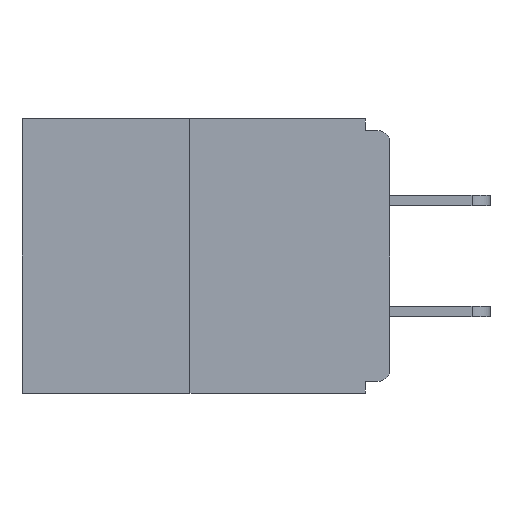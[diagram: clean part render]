
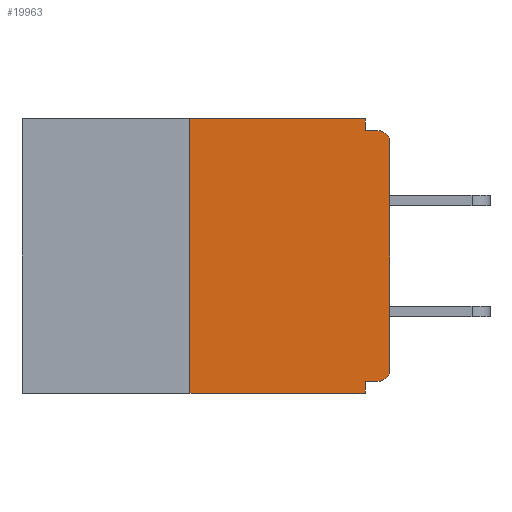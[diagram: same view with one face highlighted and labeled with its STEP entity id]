
A CAD part, left-side view. The second image highlights one B-rep face of the part: STEP entity #19963.
In plain terms, the highlighted planar face has unit normal (-1, 0, 0).
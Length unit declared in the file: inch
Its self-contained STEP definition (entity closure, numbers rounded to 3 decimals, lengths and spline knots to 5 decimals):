
#138 = LINE ( 'NONE', #4643, #24657 ) ;
#224 = AXIS2_PLACEMENT_3D ( 'NONE', #18330, #16523, #4364 ) ;
#306 = CARTESIAN_POINT ( 'NONE',  ( 0., 0.015, -0.015 ) ) ;
#425 = VECTOR ( 'NONE', #6762, 39.37008 ) ;
#967 = CARTESIAN_POINT ( 'NONE',  ( 0., 0.031, 0. ) ) ;
#1946 = AXIS2_PLACEMENT_3D ( 'NONE', #11860, #19660, #15845 ) ;
#2314 = VECTOR ( 'NONE', #6953, 39.37008 ) ;
#3305 = CIRCLE ( 'NONE', #224, 0.015 ) ;
#3632 = CARTESIAN_POINT ( 'NONE',  ( 0., 0.25, 0. ) ) ;
#3695 = VERTEX_POINT ( 'NONE', #3632 ) ;
#3914 = CARTESIAN_POINT ( 'NONE',  ( 0., 0.015, -0.328 ) ) ;
#3977 = EDGE_CURVE ( 'NONE', #23611, #12192, #20432, .T. ) ;
#4364 = DIRECTION ( 'NONE',  ( 0., 0., -1. ) ) ;
#4429 = ORIENTED_EDGE ( 'NONE', *, *, #24929, .F. ) ;
#4643 = CARTESIAN_POINT ( 'NONE',  ( 0., 0., -0.015 ) ) ;
#5482 = CARTESIAN_POINT ( 'NONE',  ( 0., 0.031, -0.015 ) ) ;
#5668 = EDGE_LOOP ( 'NONE', ( #17710, #5716, #22383, #4429, #19075, #8881, #5933, #19249, #15298, #19998 ) ) ;
#5716 = ORIENTED_EDGE ( 'NONE', *, *, #23115, .F. ) ;
#5933 = ORIENTED_EDGE ( 'NONE', *, *, #22079, .T. ) ;
#5992 = EDGE_CURVE ( 'NONE', #10187, #15060, #15591, .T. ) ;
#6681 = DIRECTION ( 'NONE',  ( 0., -1., 0. ) ) ;
#6762 = DIRECTION ( 'NONE',  ( 0., -1., 0. ) ) ;
#6953 = DIRECTION ( 'NONE',  ( 0., 1., 0. ) ) ;
#7119 = LINE ( 'NONE', #25156, #425 ) ;
#8229 = DIRECTION ( 'NONE',  ( -1., 0., 0. ) ) ;
#8346 = FACE_OUTER_BOUND ( 'NONE', #5668, .T. ) ;
#8674 = DIRECTION ( 'NONE',  ( 0., 0., 1. ) ) ;
#8881 = ORIENTED_EDGE ( 'NONE', *, *, #19013, .T. ) ;
#8905 = CARTESIAN_POINT ( 'NONE',  ( 0., 0., -0.328 ) ) ;
#9274 = CARTESIAN_POINT ( 'NONE',  ( 0., 0., -0.03 ) ) ;
#10022 = CARTESIAN_POINT ( 'NONE',  ( 0., 0.25, -0.343 ) ) ;
#10187 = VERTEX_POINT ( 'NONE', #9274 ) ;
#10892 = EDGE_CURVE ( 'NONE', #13697, #20250, #13803, .T. ) ;
#11008 = CARTESIAN_POINT ( 'NONE',  ( 0., 0., 0. ) ) ;
#11817 = CARTESIAN_POINT ( 'NONE',  ( 0., 0.031, 0. ) ) ;
#11860 = CARTESIAN_POINT ( 'NONE',  ( 0., 0.46, 0. ) ) ;
#12050 = VECTOR ( 'NONE', #12656, 39.37008 ) ;
#12128 = AXIS2_PLACEMENT_3D ( 'NONE', #18257, #8229, #24152 ) ;
#12192 = VERTEX_POINT ( 'NONE', #5482 ) ;
#12656 = DIRECTION ( 'NONE',  ( 0., 0., 1. ) ) ;
#13367 = VECTOR ( 'NONE', #8674, 39.37008 ) ;
#13697 = VERTEX_POINT ( 'NONE', #3914 ) ;
#13698 = PLANE ( 'NONE',  #1946 ) ;
#13803 = LINE ( 'NONE', #8905, #2314 ) ;
#15060 = VERTEX_POINT ( 'NONE', #306 ) ;
#15298 = ORIENTED_EDGE ( 'NONE', *, *, #26276, .F. ) ;
#15591 = CIRCLE ( 'NONE', #12128, 0.015 ) ;
#15766 = VECTOR ( 'NONE', #22341, 39.37008 ) ;
#15845 = DIRECTION ( 'NONE',  ( 0., 0., -1. ) ) ;
#16206 = LINE ( 'NONE', #11008, #13367 ) ;
#16388 = LINE ( 'NONE', #24150, #15766 ) ;
#16523 = DIRECTION ( 'NONE',  ( -1., 0., 0. ) ) ;
#16719 = CARTESIAN_POINT ( 'NONE',  ( 0., 0.25, 0. ) ) ;
#17710 = ORIENTED_EDGE ( 'NONE', *, *, #19115, .F. ) ;
#18257 = CARTESIAN_POINT ( 'NONE',  ( 0., 0.015, -0.03 ) ) ;
#18330 = CARTESIAN_POINT ( 'NONE',  ( 0., 0.015, -0.313 ) ) ;
#18828 = CARTESIAN_POINT ( 'NONE',  ( 0., 0.031, -0.343 ) ) ;
#19013 = EDGE_CURVE ( 'NONE', #13697, #20844, #3305, .T. ) ;
#19042 = CARTESIAN_POINT ( 'NONE',  ( 0., 0., -0.313 ) ) ;
#19075 = ORIENTED_EDGE ( 'NONE', *, *, #10892, .F. ) ;
#19115 = EDGE_CURVE ( 'NONE', #3695, #23611, #7119, .T. ) ;
#19249 = ORIENTED_EDGE ( 'NONE', *, *, #5992, .T. ) ;
#19660 = DIRECTION ( 'NONE',  ( 1., 0., 0. ) ) ;
#19792 = VECTOR ( 'NONE', #24338, 39.37008 ) ;
#19963 = ADVANCED_FACE ( 'NONE', ( #8346 ), #13698, .F. ) ;
#19998 = ORIENTED_EDGE ( 'NONE', *, *, #3977, .F. ) ;
#20250 = VERTEX_POINT ( 'NONE', #22997 ) ;
#20432 = LINE ( 'NONE', #11817, #19792 ) ;
#20664 = VERTEX_POINT ( 'NONE', #10022 ) ;
#20844 = VERTEX_POINT ( 'NONE', #19042 ) ;
#20860 = VECTOR ( 'NONE', #21722, 39.37008 ) ;
#21722 = DIRECTION ( 'NONE',  ( 0., -1., 0. ) ) ;
#22079 = EDGE_CURVE ( 'NONE', #20844, #10187, #16206, .T. ) ;
#22341 = DIRECTION ( 'NONE',  ( 0., 0., -1. ) ) ;
#22383 = ORIENTED_EDGE ( 'NONE', *, *, #24678, .T. ) ;
#22835 = LINE ( 'NONE', #16719, #12050 ) ;
#22997 = CARTESIAN_POINT ( 'NONE',  ( 0., 0.031, -0.328 ) ) ;
#23115 = EDGE_CURVE ( 'NONE', #20664, #3695, #22835, .T. ) ;
#23611 = VERTEX_POINT ( 'NONE', #967 ) ;
#23735 = LINE ( 'NONE', #25574, #20860 ) ;
#24150 = CARTESIAN_POINT ( 'NONE',  ( 0., 0.031, -0.343 ) ) ;
#24152 = DIRECTION ( 'NONE',  ( 0., 0., -1. ) ) ;
#24338 = DIRECTION ( 'NONE',  ( 0., 0., -1. ) ) ;
#24657 = VECTOR ( 'NONE', #6681, 39.37008 ) ;
#24678 = EDGE_CURVE ( 'NONE', #20664, #25430, #23735, .T. ) ;
#24929 = EDGE_CURVE ( 'NONE', #20250, #25430, #16388, .T. ) ;
#25156 = CARTESIAN_POINT ( 'NONE',  ( 0., 0.46, 0. ) ) ;
#25430 = VERTEX_POINT ( 'NONE', #18828 ) ;
#25574 = CARTESIAN_POINT ( 'NONE',  ( 0., 0.46, -0.343 ) ) ;
#26276 = EDGE_CURVE ( 'NONE', #12192, #15060, #138, .T. ) ;
